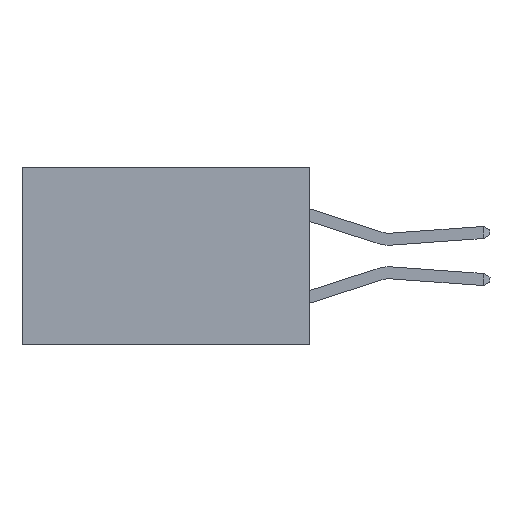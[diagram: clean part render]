
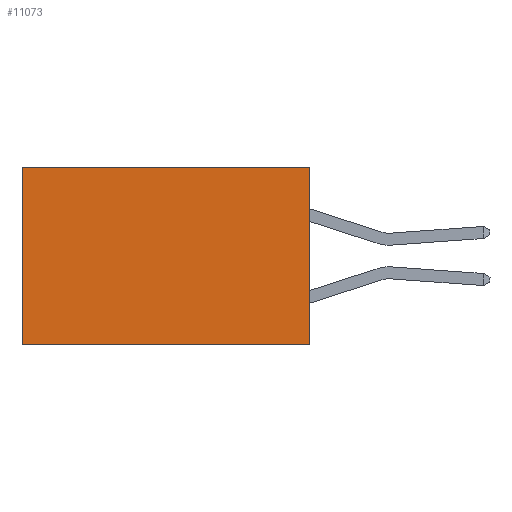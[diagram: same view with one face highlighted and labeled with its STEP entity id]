
A CAD part, left-side view. The second image highlights one B-rep face of the part: STEP entity #11073.
In plain terms, the highlighted planar face has unit normal (-1, 0, 0).
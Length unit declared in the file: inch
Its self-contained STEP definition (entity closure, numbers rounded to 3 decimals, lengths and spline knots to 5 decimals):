
#149 = AXIS2_PLACEMENT_3D ( 'NONE', #14437, #5869, #15842 ) ;
#290 = VECTOR ( 'NONE', #6819, 39.37008 ) ;
#1751 = CARTESIAN_POINT ( 'NONE',  ( 0.2615, 0., -0.37 ) ) ;
#3224 = VECTOR ( 'NONE', #18588, 39.37008 ) ;
#3581 = CARTESIAN_POINT ( 'NONE',  ( 0.2615, 0., -0.37 ) ) ;
#4138 = FACE_OUTER_BOUND ( 'NONE', #6118, .T. ) ;
#4399 = PLANE ( 'NONE',  #149 ) ;
#4576 = LINE ( 'NONE', #1751, #7963 ) ;
#5380 = CARTESIAN_POINT ( 'NONE',  ( 0.2615, 0.6, -0.37 ) ) ;
#5477 = VECTOR ( 'NONE', #18024, 39.37008 ) ;
#5869 = DIRECTION ( 'NONE',  ( 1., 0., 0. ) ) ;
#6118 = EDGE_LOOP ( 'NONE', ( #17384, #17369, #6982, #11274 ) ) ;
#6451 = EDGE_CURVE ( 'NONE', #12376, #17714, #4576, .T. ) ;
#6819 = DIRECTION ( 'NONE',  ( 0., 0., -1. ) ) ;
#6982 = ORIENTED_EDGE ( 'NONE', *, *, #6451, .F. ) ;
#7115 = LINE ( 'NONE', #7311, #3224 ) ;
#7218 = EDGE_CURVE ( 'NONE', #17714, #14194, #9280, .T. ) ;
#7311 = CARTESIAN_POINT ( 'NONE',  ( 0.2615, 0., 0. ) ) ;
#7963 = VECTOR ( 'NONE', #11886, 39.37008 ) ;
#8564 = VERTEX_POINT ( 'NONE', #16160 ) ;
#8878 = EDGE_CURVE ( 'NONE', #8564, #14194, #11901, .T. ) ;
#9280 = LINE ( 'NONE', #10938, #5477 ) ;
#10938 = CARTESIAN_POINT ( 'NONE',  ( 0.2615, 0., -0.37 ) ) ;
#11073 = ADVANCED_FACE ( 'NONE', ( #4138 ), #4399, .F. ) ;
#11080 = EDGE_CURVE ( 'NONE', #12376, #8564, #7115, .T. ) ;
#11274 = ORIENTED_EDGE ( 'NONE', *, *, #11080, .T. ) ;
#11886 = DIRECTION ( 'NONE',  ( 0., 0., -1. ) ) ;
#11901 = LINE ( 'NONE', #5380, #290 ) ;
#12376 = VERTEX_POINT ( 'NONE', #15382 ) ;
#13540 = CARTESIAN_POINT ( 'NONE',  ( 0.2615, 0.6, -0.37 ) ) ;
#14194 = VERTEX_POINT ( 'NONE', #13540 ) ;
#14437 = CARTESIAN_POINT ( 'NONE',  ( 0.2615, 0., -0.37 ) ) ;
#15382 = CARTESIAN_POINT ( 'NONE',  ( 0.2615, 0., 0. ) ) ;
#15842 = DIRECTION ( 'NONE',  ( 0., 0., -1. ) ) ;
#16160 = CARTESIAN_POINT ( 'NONE',  ( 0.2615, 0.6, 0. ) ) ;
#17369 = ORIENTED_EDGE ( 'NONE', *, *, #7218, .F. ) ;
#17384 = ORIENTED_EDGE ( 'NONE', *, *, #8878, .T. ) ;
#17714 = VERTEX_POINT ( 'NONE', #3581 ) ;
#18024 = DIRECTION ( 'NONE',  ( 0., 1., 0. ) ) ;
#18588 = DIRECTION ( 'NONE',  ( 0., 1., 0. ) ) ;
